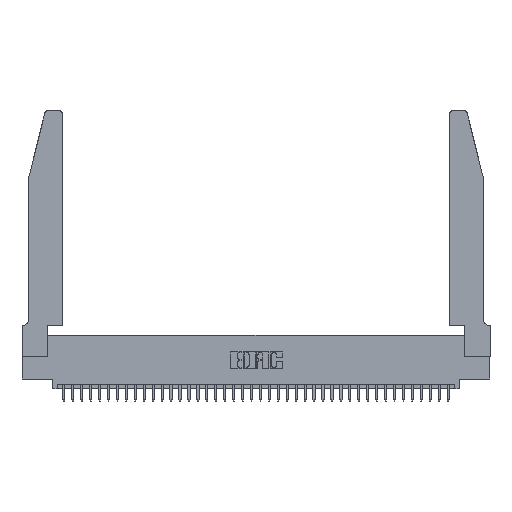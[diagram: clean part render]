
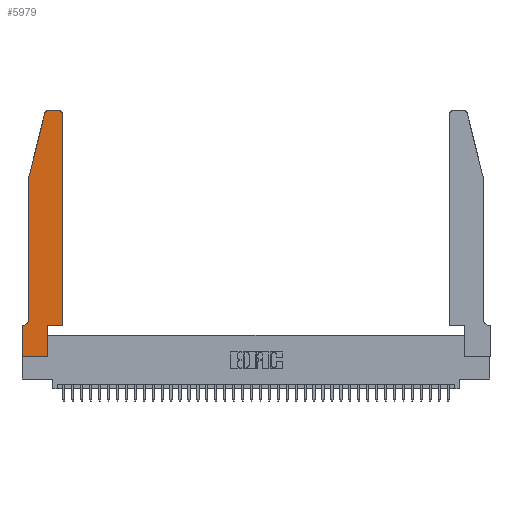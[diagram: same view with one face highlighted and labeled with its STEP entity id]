
A CAD part, top view. The second image highlights one B-rep face of the part: STEP entity #5979.
In plain terms, the highlighted planar face has unit normal (0, 0, 1).
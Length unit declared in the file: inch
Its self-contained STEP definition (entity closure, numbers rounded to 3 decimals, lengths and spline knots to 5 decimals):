
#326 = DIRECTION ( 'NONE',  ( 0., 0., 1. ) ) ;
#797 = ORIENTED_EDGE ( 'NONE', *, *, #26627, .T. ) ;
#1049 = CARTESIAN_POINT ( 'NONE',  ( 0.4505, 0.35, 0.37 ) ) ;
#1080 = EDGE_LOOP ( 'NONE', ( #36186, #33321, #15757, #797, #28631, #38342, #8319, #11126, #18107, #24537, #37244, #33102 ) ) ;
#1797 = VERTEX_POINT ( 'NONE', #12472 ) ;
#2616 = EDGE_CURVE ( 'NONE', #14763, #14019, #38034, .T. ) ;
#3170 = VECTOR ( 'NONE', #37252, 39.37008 ) ;
#3315 = VECTOR ( 'NONE', #6359, 39.37008 ) ;
#3434 = DIRECTION ( 'NONE',  ( 0., -1., 0. ) ) ;
#4532 = CARTESIAN_POINT ( 'NONE',  ( 0.4505, 0.35, 0.37 ) ) ;
#5108 = VERTEX_POINT ( 'NONE', #11239 ) ;
#5540 = VERTEX_POINT ( 'NONE', #37269 ) ;
#5772 = VECTOR ( 'NONE', #3434, 39.37008 ) ;
#5979 = ADVANCED_FACE ( 'NONE', ( #10476 ), #9609, .T. ) ;
#6359 = DIRECTION ( 'NONE',  ( 0., -1., 0. ) ) ;
#6432 = VECTOR ( 'NONE', #17542, 39.37008 ) ;
#6716 = AXIS2_PLACEMENT_3D ( 'NONE', #27535, #326, #21665 ) ;
#7309 = CARTESIAN_POINT ( 'NONE',  ( 0.2865, 0.35, 0.37 ) ) ;
#7678 = DIRECTION ( 'NONE',  ( 0., 1., 0. ) ) ;
#7753 = CARTESIAN_POINT ( 'NONE',  ( 0.284, 2.75, 0.37 ) ) ;
#8207 = AXIS2_PLACEMENT_3D ( 'NONE', #13207, #34182, #16219 ) ;
#8319 = ORIENTED_EDGE ( 'NONE', *, *, #16717, .T. ) ;
#8382 = EDGE_CURVE ( 'NONE', #14019, #34671, #30984, .T. ) ;
#8429 = VERTEX_POINT ( 'NONE', #7309 ) ;
#9609 = PLANE ( 'NONE',  #6716 ) ;
#10131 = DIRECTION ( 'NONE',  ( -1., 0., 0. ) ) ;
#10476 = FACE_OUTER_BOUND ( 'NONE', #1080, .T. ) ;
#10676 = LINE ( 'NONE', #1049, #32722 ) ;
#11126 = ORIENTED_EDGE ( 'NONE', *, *, #30936, .T. ) ;
#11239 = CARTESIAN_POINT ( 'NONE',  ( 0.0755, 0.42, 0.37 ) ) ;
#11996 = LINE ( 'NONE', #30653, #5772 ) ;
#12472 = CARTESIAN_POINT ( 'NONE',  ( 0., 0.35, 0.37 ) ) ;
#12488 = CARTESIAN_POINT ( 'NONE',  ( 0., 0., 0.37 ) ) ;
#12572 = DIRECTION ( 'NONE',  ( 0., 0., -1. ) ) ;
#12614 = CARTESIAN_POINT ( 'NONE',  ( 0.0755, 0.35, 0.37 ) ) ;
#13113 = CARTESIAN_POINT ( 'NONE',  ( 0.2865, 0., 0.37 ) ) ;
#13207 = CARTESIAN_POINT ( 'NONE',  ( 0.4205, 2.72, 0.37 ) ) ;
#13267 = CARTESIAN_POINT ( 'NONE',  ( 0.0755, 2., 0.37 ) ) ;
#13566 = VECTOR ( 'NONE', #24638, 39.37008 ) ;
#14019 = VERTEX_POINT ( 'NONE', #15077 ) ;
#14176 = VERTEX_POINT ( 'NONE', #34038 ) ;
#14763 = VERTEX_POINT ( 'NONE', #16041 ) ;
#15061 = VECTOR ( 'NONE', #10131, 39.37008 ) ;
#15077 = CARTESIAN_POINT ( 'NONE',  ( 0.4205, 2.75, 0.37 ) ) ;
#15297 = VERTEX_POINT ( 'NONE', #13113 ) ;
#15582 = CARTESIAN_POINT ( 'NONE',  ( 0.284, 2.72, 0.37 ) ) ;
#15620 = CARTESIAN_POINT ( 'NONE',  ( 0., 0., 0.37 ) ) ;
#15757 = ORIENTED_EDGE ( 'NONE', *, *, #35216, .T. ) ;
#16041 = CARTESIAN_POINT ( 'NONE',  ( 0.4505, 2.72, 0.37 ) ) ;
#16219 = DIRECTION ( 'NONE',  ( 1., 0., 0. ) ) ;
#16717 = EDGE_CURVE ( 'NONE', #1797, #14176, #35479, .T. ) ;
#17542 = DIRECTION ( 'NONE',  ( 0., 1., 0. ) ) ;
#18107 = ORIENTED_EDGE ( 'NONE', *, *, #31392, .T. ) ;
#18396 = VERTEX_POINT ( 'NONE', #38314 ) ;
#18551 = DIRECTION ( 'NONE',  ( 1., 0., 0. ) ) ;
#19049 = EDGE_CURVE ( 'NONE', #5540, #1797, #24653, .T. ) ;
#19109 = VERTEX_POINT ( 'NONE', #36749 ) ;
#19304 = DIRECTION ( 'NONE',  ( 1., 0., 0. ) ) ;
#20313 = LINE ( 'NONE', #13267, #3170 ) ;
#21665 = DIRECTION ( 'NONE',  ( 1., 0., 0. ) ) ;
#22417 = LINE ( 'NONE', #4532, #38382 ) ;
#23736 = VECTOR ( 'NONE', #27534, 39.37008 ) ;
#24537 = ORIENTED_EDGE ( 'NONE', *, *, #25548, .T. ) ;
#24638 = DIRECTION ( 'NONE',  ( 1., 0., 0. ) ) ;
#24653 = LINE ( 'NONE', #12614, #23736 ) ;
#25548 = EDGE_CURVE ( 'NONE', #8429, #18396, #10676, .T. ) ;
#26627 = EDGE_CURVE ( 'NONE', #19109, #5108, #11996, .T. ) ;
#27204 = AXIS2_PLACEMENT_3D ( 'NONE', #15582, #36563, #18551 ) ;
#27534 = DIRECTION ( 'NONE',  ( -1., 0., 0. ) ) ;
#27535 = CARTESIAN_POINT ( 'NONE',  ( 0., 0.35, 0.37 ) ) ;
#27933 = CARTESIAN_POINT ( 'NONE',  ( 0.2605, 2.75, 0.37 ) ) ;
#28631 = ORIENTED_EDGE ( 'NONE', *, *, #35741, .T. ) ;
#30208 = VERTEX_POINT ( 'NONE', #32708 ) ;
#30436 = LINE ( 'NONE', #32503, #6432 ) ;
#30520 = CARTESIAN_POINT ( 'NONE',  ( 0.0055, 0.42, 0.37 ) ) ;
#30653 = CARTESIAN_POINT ( 'NONE',  ( 0.0755, 2., 0.37 ) ) ;
#30936 = EDGE_CURVE ( 'NONE', #14176, #15297, #36591, .T. ) ;
#30984 = LINE ( 'NONE', #27933, #15061 ) ;
#31187 = EDGE_CURVE ( 'NONE', #18396, #14763, #22417, .T. ) ;
#31392 = EDGE_CURVE ( 'NONE', #15297, #8429, #30436, .T. ) ;
#31625 = EDGE_CURVE ( 'NONE', #34671, #30208, #37925, .T. ) ;
#32503 = CARTESIAN_POINT ( 'NONE',  ( 0.2865, 0.35, 0.37 ) ) ;
#32708 = CARTESIAN_POINT ( 'NONE',  ( 0.25487, 2.72718, 0.37 ) ) ;
#32722 = VECTOR ( 'NONE', #19304, 39.37008 ) ;
#33102 = ORIENTED_EDGE ( 'NONE', *, *, #2616, .T. ) ;
#33321 = ORIENTED_EDGE ( 'NONE', *, *, #31625, .T. ) ;
#33394 = CIRCLE ( 'NONE', #36374, 0.07 ) ;
#33551 = DIRECTION ( 'NONE',  ( -1., 0., 0. ) ) ;
#34038 = CARTESIAN_POINT ( 'NONE',  ( 0., 0., 0.37 ) ) ;
#34182 = DIRECTION ( 'NONE',  ( 0., 0., 1. ) ) ;
#34671 = VERTEX_POINT ( 'NONE', #7753 ) ;
#35216 = EDGE_CURVE ( 'NONE', #30208, #19109, #20313, .T. ) ;
#35479 = LINE ( 'NONE', #12488, #3315 ) ;
#35741 = EDGE_CURVE ( 'NONE', #5108, #5540, #33394, .T. ) ;
#36186 = ORIENTED_EDGE ( 'NONE', *, *, #8382, .T. ) ;
#36374 = AXIS2_PLACEMENT_3D ( 'NONE', #30520, #12572, #33551 ) ;
#36563 = DIRECTION ( 'NONE',  ( 0., 0., 1. ) ) ;
#36591 = LINE ( 'NONE', #15620, #13566 ) ;
#36749 = CARTESIAN_POINT ( 'NONE',  ( 0.0755, 2., 0.37 ) ) ;
#37244 = ORIENTED_EDGE ( 'NONE', *, *, #31187, .T. ) ;
#37252 = DIRECTION ( 'NONE',  ( -0.239, -0.971, 0. ) ) ;
#37269 = CARTESIAN_POINT ( 'NONE',  ( 0.0055, 0.35, 0.37 ) ) ;
#37925 = CIRCLE ( 'NONE', #27204, 0.03 ) ;
#38034 = CIRCLE ( 'NONE', #8207, 0.03 ) ;
#38314 = CARTESIAN_POINT ( 'NONE',  ( 0.4505, 0.35, 0.37 ) ) ;
#38342 = ORIENTED_EDGE ( 'NONE', *, *, #19049, .T. ) ;
#38382 = VECTOR ( 'NONE', #7678, 39.37008 ) ;
